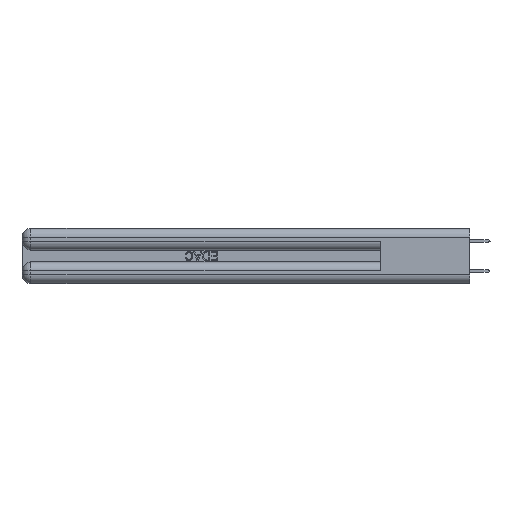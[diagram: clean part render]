
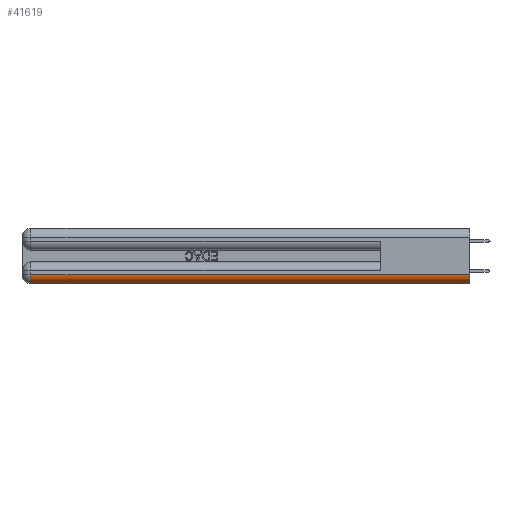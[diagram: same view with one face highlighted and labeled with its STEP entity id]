
A CAD part, left-side view. The second image highlights one B-rep face of the part: STEP entity #41619.
In plain terms, the highlighted cylindrical face has radius 1.524 mm (diameter 3.048 mm), a partial arc.
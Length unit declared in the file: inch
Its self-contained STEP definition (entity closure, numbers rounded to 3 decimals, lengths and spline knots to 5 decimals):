
#366 = DIRECTION ( 'NONE',  ( 0., 1., 0. ) ) ;
#2987 = LINE ( 'NONE', #30622, #39925 ) ;
#3489 = FACE_OUTER_BOUND ( 'NONE', #13293, .T. ) ;
#6658 = EDGE_CURVE ( 'NONE', #43722, #8436, #7611, .T. ) ;
#7394 = CIRCLE ( 'NONE', #8865, 0.06 ) ;
#7611 = LINE ( 'NONE', #24585, #11953 ) ;
#8436 = VERTEX_POINT ( 'NONE', #43103 ) ;
#8865 = AXIS2_PLACEMENT_3D ( 'NONE', #14886, #15337, #25328 ) ;
#11953 = VECTOR ( 'NONE', #366, 39.37008 ) ;
#13293 = EDGE_LOOP ( 'NONE', ( #30927, #35826, #19035, #25357 ) ) ;
#14886 = CARTESIAN_POINT ( 'NONE',  ( 0.06, 0., 0.06 ) ) ;
#15337 = DIRECTION ( 'NONE',  ( 0., -1., 0. ) ) ;
#15799 = DIRECTION ( 'NONE',  ( 0., 1., 0. ) ) ;
#17500 = DIRECTION ( 'NONE',  ( 0., 0., 1. ) ) ;
#18124 = EDGE_CURVE ( 'NONE', #8436, #32813, #34101, .T. ) ;
#18998 = DIRECTION ( 'NONE',  ( 0., 0., 1. ) ) ;
#19035 = ORIENTED_EDGE ( 'NONE', *, *, #18124, .F. ) ;
#23298 = CARTESIAN_POINT ( 'NONE',  ( 0., 2.94, 0.06 ) ) ;
#24585 = CARTESIAN_POINT ( 'NONE',  ( 0.06, 3., 0. ) ) ;
#25328 = DIRECTION ( 'NONE',  ( 0., 0., 1. ) ) ;
#25357 = ORIENTED_EDGE ( 'NONE', *, *, #6658, .F. ) ;
#27495 = DIRECTION ( 'NONE',  ( 0., 1., 0. ) ) ;
#28150 = CARTESIAN_POINT ( 'NONE',  ( 0.06, 0., 0.06 ) ) ;
#28585 = EDGE_CURVE ( 'NONE', #32813, #43375, #2987, .T. ) ;
#30622 = CARTESIAN_POINT ( 'NONE',  ( 0., 0., 0.06 ) ) ;
#30927 = ORIENTED_EDGE ( 'NONE', *, *, #38266, .F. ) ;
#31562 = CYLINDRICAL_SURFACE ( 'NONE', #32899, 0.06 ) ;
#32813 = VERTEX_POINT ( 'NONE', #23298 ) ;
#32899 = AXIS2_PLACEMENT_3D ( 'NONE', #28150, #27495, #17500 ) ;
#34101 = CIRCLE ( 'NONE', #42760, 0.06 ) ;
#35826 = ORIENTED_EDGE ( 'NONE', *, *, #28585, .F. ) ;
#36930 = CARTESIAN_POINT ( 'NONE',  ( 0., 0., 0.06 ) ) ;
#38266 = EDGE_CURVE ( 'NONE', #43375, #43722, #7394, .T. ) ;
#39818 = CARTESIAN_POINT ( 'NONE',  ( 0.06, 2.94, 0.06 ) ) ;
#39925 = VECTOR ( 'NONE', #44440, 39.37008 ) ;
#41619 = ADVANCED_FACE ( 'NONE', ( #3489 ), #31562, .T. ) ;
#42760 = AXIS2_PLACEMENT_3D ( 'NONE', #39818, #15799, #18998 ) ;
#43012 = CARTESIAN_POINT ( 'NONE',  ( 0.06, 0., 0. ) ) ;
#43103 = CARTESIAN_POINT ( 'NONE',  ( 0.06, 2.94, 0. ) ) ;
#43375 = VERTEX_POINT ( 'NONE', #36930 ) ;
#43722 = VERTEX_POINT ( 'NONE', #43012 ) ;
#44440 = DIRECTION ( 'NONE',  ( 0., -1., 0. ) ) ;
